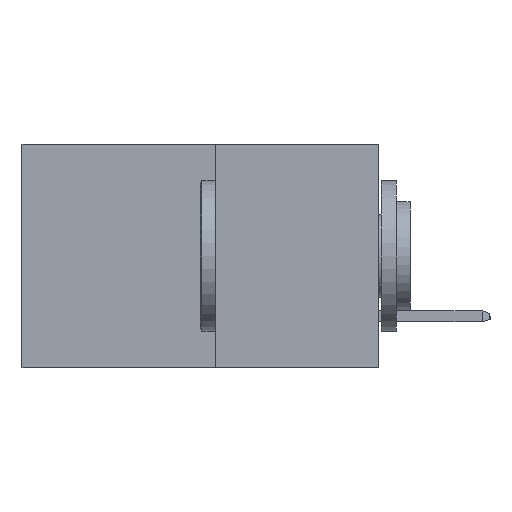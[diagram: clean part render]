
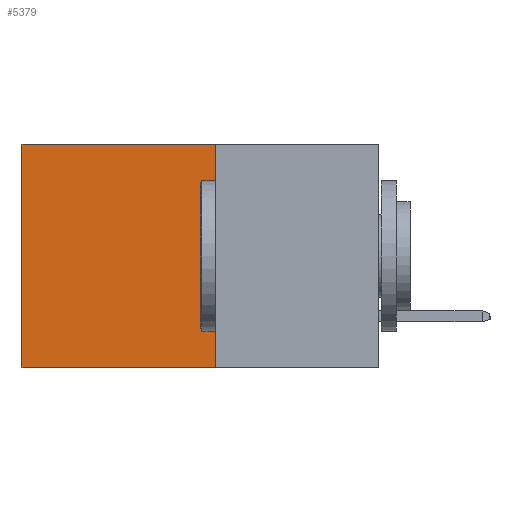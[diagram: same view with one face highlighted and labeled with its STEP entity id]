
A CAD part, left-side view. The second image highlights one B-rep face of the part: STEP entity #5379.
In plain terms, the highlighted planar face has unit normal (-1, 0, 0).
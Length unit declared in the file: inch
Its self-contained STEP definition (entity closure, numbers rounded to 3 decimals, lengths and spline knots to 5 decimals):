
#2001 = LINE ( 'NONE', #13869, #10772 ) ;
#2412 = CARTESIAN_POINT ( 'NONE',  ( 0.277, 0.27, -0.37 ) ) ;
#2616 = LINE ( 'NONE', #14314, #11700 ) ;
#3131 = DIRECTION ( 'NONE',  ( 0., 0., -1. ) ) ;
#3303 = DIRECTION ( 'NONE',  ( 0., 0., -1. ) ) ;
#4026 = EDGE_CURVE ( 'NONE', #13090, #12536, #2616, .T. ) ;
#4052 = ORIENTED_EDGE ( 'NONE', *, *, #7334, .F. ) ;
#4068 = VERTEX_POINT ( 'NONE', #13848 ) ;
#4188 = FACE_OUTER_BOUND ( 'NONE', #4601, .T. ) ;
#4601 = EDGE_LOOP ( 'NONE', ( #6751, #9764, #4052, #10130 ) ) ;
#5379 = ADVANCED_FACE ( 'NONE', ( #4188 ), #8795, .F. ) ;
#6016 = EDGE_CURVE ( 'NONE', #4068, #7580, #2001, .T. ) ;
#6751 = ORIENTED_EDGE ( 'NONE', *, *, #10669, .T. ) ;
#6946 = CARTESIAN_POINT ( 'NONE',  ( 0.277, 0.59, 0. ) ) ;
#7334 = EDGE_CURVE ( 'NONE', #4068, #13090, #11421, .T. ) ;
#7580 = VERTEX_POINT ( 'NONE', #6946 ) ;
#7697 = LINE ( 'NONE', #10136, #10374 ) ;
#8634 = DIRECTION ( 'NONE',  ( 0., 0., -1. ) ) ;
#8679 = DIRECTION ( 'NONE',  ( 1., 0., 0. ) ) ;
#8795 = PLANE ( 'NONE',  #8863 ) ;
#8842 = CARTESIAN_POINT ( 'NONE',  ( 0.277, 0.27, -0.37 ) ) ;
#8863 = AXIS2_PLACEMENT_3D ( 'NONE', #8901, #8679, #8634 ) ;
#8901 = CARTESIAN_POINT ( 'NONE',  ( 0.277, 0.27, -0.37 ) ) ;
#9764 = ORIENTED_EDGE ( 'NONE', *, *, #4026, .F. ) ;
#10130 = ORIENTED_EDGE ( 'NONE', *, *, #6016, .T. ) ;
#10136 = CARTESIAN_POINT ( 'NONE',  ( 0.277, 0.59, -0.37 ) ) ;
#10374 = VECTOR ( 'NONE', #3303, 39.37008 ) ;
#10540 = CARTESIAN_POINT ( 'NONE',  ( 0.277, 0.59, -0.37 ) ) ;
#10669 = EDGE_CURVE ( 'NONE', #7580, #12536, #7697, .T. ) ;
#10772 = VECTOR ( 'NONE', #14158, 39.37008 ) ;
#11421 = LINE ( 'NONE', #8842, #11787 ) ;
#11700 = VECTOR ( 'NONE', #14403, 39.37008 ) ;
#11787 = VECTOR ( 'NONE', #3131, 39.37008 ) ;
#12536 = VERTEX_POINT ( 'NONE', #10540 ) ;
#13090 = VERTEX_POINT ( 'NONE', #2412 ) ;
#13848 = CARTESIAN_POINT ( 'NONE',  ( 0.277, 0.27, 0. ) ) ;
#13869 = CARTESIAN_POINT ( 'NONE',  ( 0.277, 0.27, 0. ) ) ;
#14158 = DIRECTION ( 'NONE',  ( 0., 1., 0. ) ) ;
#14314 = CARTESIAN_POINT ( 'NONE',  ( 0.277, 0.27, -0.37 ) ) ;
#14403 = DIRECTION ( 'NONE',  ( 0., 1., 0. ) ) ;
